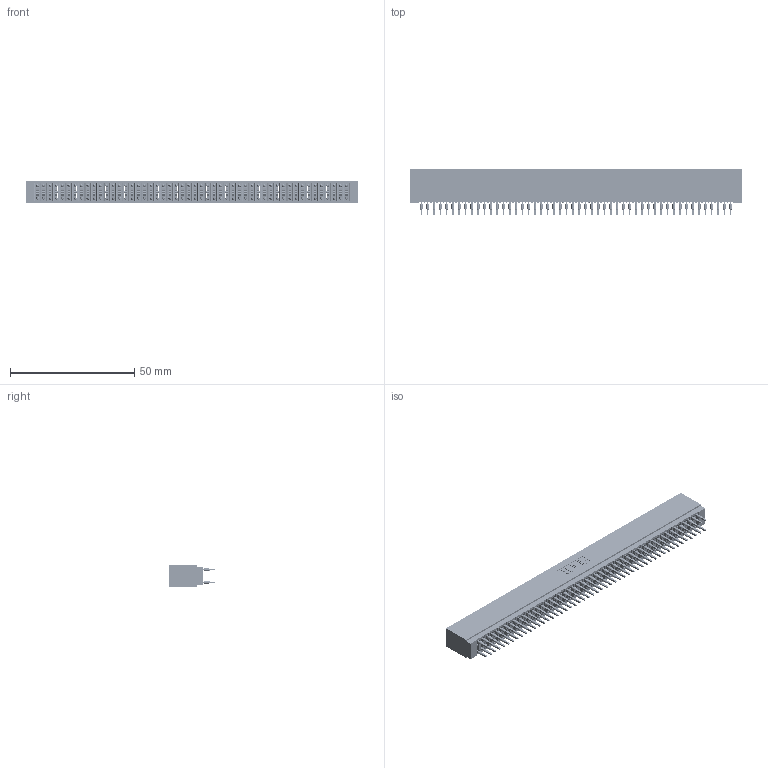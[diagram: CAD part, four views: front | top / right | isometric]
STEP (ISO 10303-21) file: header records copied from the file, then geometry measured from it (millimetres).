
FILE_DESCRIPTION (( 'STEP AP203' ), '1' );
FILE_NAME ('725-100-560-201.STEP', '2026-02-24T20:00:36', ( '' ), ( '' ), 'SwSTEP 2.0', 'SolidWorks 2023', '' );
FILE_SCHEMA (( 'CONFIG_CONTROL_DESIGN' ));
Length unit declared in the file: millimetre
Products named in the file (3): 745-292-001_560; 725-100-560-201; 725 Part_Insulator Option - 01
Assembly tree (101 placements, depth 2):
  725-100-560-201
    725 Part_Insulator Option - 01
    745-292-001_560  x100
Bounding box: 133.6 x 18.8 x 8.89 mm (x, y, z)
Volume: 10924 mm3; surface area: 24820.8 mm2
Topology: 101 solids, 101 shells, 9945 faces, 27204 edges, 17268 vertices
Faces by surface type: plane 5155, cylinder 2190, bspline 2000, torus 600
Entity records: 83371 total; most frequent: CARTESIAN_POINT 14961, ORIENTED_EDGE 14412, DIRECTION 12590, EDGE_CURVE 7206, VECTOR 6716, LINE 6716, VERTEX_POINT 4596, AXIS2_PLACEMENT_3D 2937
